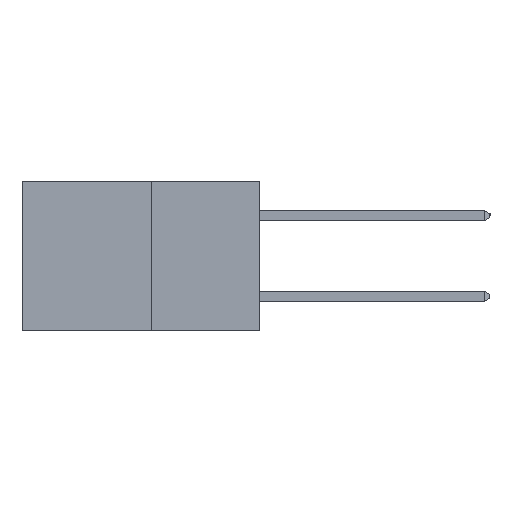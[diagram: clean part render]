
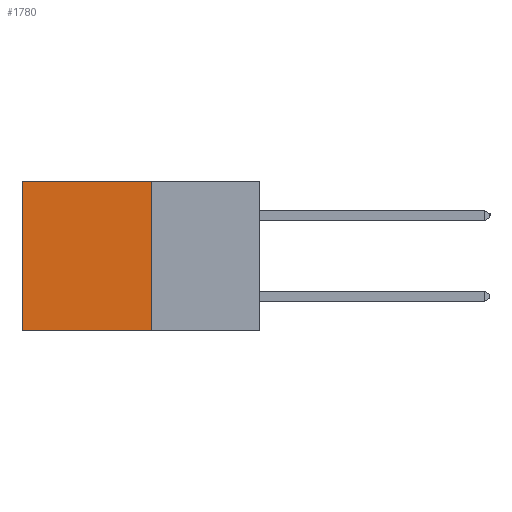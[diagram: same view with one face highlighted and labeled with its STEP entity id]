
A CAD part, left-side view. The second image highlights one B-rep face of the part: STEP entity #1780.
In plain terms, the highlighted planar face has unit normal (-1, 0, 0).
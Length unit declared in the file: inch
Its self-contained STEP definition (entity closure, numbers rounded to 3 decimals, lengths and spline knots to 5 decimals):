
#285 = DIRECTION ( 'NONE',  ( 0., 0., -1. ) ) ;
#307 = CARTESIAN_POINT ( 'NONE',  ( 0.277, 0.59, -0.37 ) ) ;
#753 = CARTESIAN_POINT ( 'NONE',  ( 0.277, 0.59, -0.37 ) ) ;
#1012 = AXIS2_PLACEMENT_3D ( 'NONE', #2229, #1972, #1160 ) ;
#1160 = DIRECTION ( 'NONE',  ( 0., 0., -1. ) ) ;
#1780 = ADVANCED_FACE ( 'NONE', ( #9154 ), #2004, .F. ) ;
#1972 = DIRECTION ( 'NONE',  ( 1., 0., 0. ) ) ;
#2004 = PLANE ( 'NONE',  #1012 ) ;
#2197 = ORIENTED_EDGE ( 'NONE', *, *, #5466, .F. ) ;
#2229 = CARTESIAN_POINT ( 'NONE',  ( 0.277, 0.27, -0.37 ) ) ;
#2259 = EDGE_CURVE ( 'NONE', #8521, #8379, #7256, .T. ) ;
#2260 = CARTESIAN_POINT ( 'NONE',  ( 0.277, 0.27, -0.37 ) ) ;
#2440 = VERTEX_POINT ( 'NONE', #753 ) ;
#3134 = VECTOR ( 'NONE', #3910, 39.37008 ) ;
#3563 = LINE ( 'NONE', #307, #9232 ) ;
#3782 = EDGE_CURVE ( 'NONE', #5435, #2440, #3563, .T. ) ;
#3834 = ORIENTED_EDGE ( 'NONE', *, *, #2259, .F. ) ;
#3910 = DIRECTION ( 'NONE',  ( 0., 1., 0. ) ) ;
#4017 = CARTESIAN_POINT ( 'NONE',  ( 0.277, 0.27, -0.37 ) ) ;
#4041 = ORIENTED_EDGE ( 'NONE', *, *, #6455, .T. ) ;
#4184 = CARTESIAN_POINT ( 'NONE',  ( 0.277, 0.59, 0. ) ) ;
#4399 = EDGE_LOOP ( 'NONE', ( #6761, #2197, #3834, #4041 ) ) ;
#4609 = CARTESIAN_POINT ( 'NONE',  ( 0.277, 0.27, -0.37 ) ) ;
#4823 = DIRECTION ( 'NONE',  ( 0., 0., -1. ) ) ;
#4824 = VECTOR ( 'NONE', #9482, 39.37008 ) ;
#5083 = LINE ( 'NONE', #4017, #3134 ) ;
#5435 = VERTEX_POINT ( 'NONE', #4184 ) ;
#5466 = EDGE_CURVE ( 'NONE', #8379, #2440, #5083, .T. ) ;
#6455 = EDGE_CURVE ( 'NONE', #8521, #5435, #6865, .T. ) ;
#6761 = ORIENTED_EDGE ( 'NONE', *, *, #3782, .T. ) ;
#6865 = LINE ( 'NONE', #8023, #4824 ) ;
#6931 = CARTESIAN_POINT ( 'NONE',  ( 0.277, 0.27, 0. ) ) ;
#7021 = VECTOR ( 'NONE', #4823, 39.37008 ) ;
#7256 = LINE ( 'NONE', #4609, #7021 ) ;
#8023 = CARTESIAN_POINT ( 'NONE',  ( 0.277, 0.27, 0. ) ) ;
#8379 = VERTEX_POINT ( 'NONE', #2260 ) ;
#8521 = VERTEX_POINT ( 'NONE', #6931 ) ;
#9154 = FACE_OUTER_BOUND ( 'NONE', #4399, .T. ) ;
#9232 = VECTOR ( 'NONE', #285, 39.37008 ) ;
#9482 = DIRECTION ( 'NONE',  ( 0., 1., 0. ) ) ;
